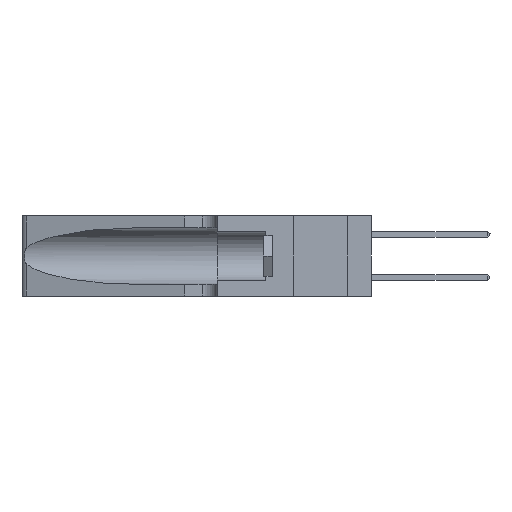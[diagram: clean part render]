
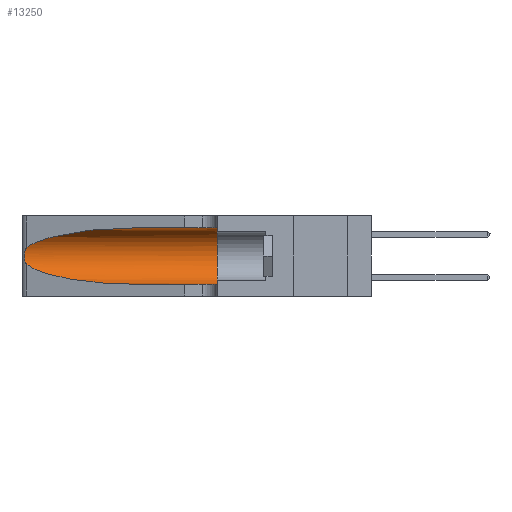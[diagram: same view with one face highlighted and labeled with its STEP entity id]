
A CAD part, left-side view. The second image highlights one B-rep face of the part: STEP entity #13250.
In plain terms, the highlighted cylindrical face has radius 3.308 mm (diameter 6.617 mm), a partial arc.
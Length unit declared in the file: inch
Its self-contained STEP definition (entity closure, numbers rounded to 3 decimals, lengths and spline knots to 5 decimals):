
#466 = DIRECTION ( 'NONE',  ( 0., -1., 0. ) ) ;
#1158 = CARTESIAN_POINT ( 'NONE',  ( 0.26018, 1.23835, 0.19895 ) ) ;
#1404 = CARTESIAN_POINT ( 'NONE',  ( 0.25487, 1.22718, 0.22369 ) ) ;
#1610 = ORIENTED_EDGE ( 'NONE', *, *, #1614, .F. ) ;
#1614 = EDGE_CURVE ( 'NONE', #12219, #10811, #5486, .T. ) ;
#2784 = VERTEX_POINT ( 'NONE', #10919 ) ;
#3236 = VERTEX_POINT ( 'NONE', #11997 ) ;
#4384 = EDGE_CURVE ( 'NONE', #2784, #16755, #19624, .T. ) ;
#5141 = DIRECTION ( 'NONE',  ( 0., 0., -1. ) ) ;
#5486 = CIRCLE ( 'NONE', #8405, 0.13025 ) ;
#5606 = CARTESIAN_POINT ( 'NONE',  ( 0.26017, 1.23833, 0.17102 ) ) ;
#5925 = CARTESIAN_POINT ( 'NONE',  ( 0.1305, 0.72297, 0.31525 ) ) ;
#6008 = ORIENTED_EDGE ( 'NONE', *, *, #16518, .T. ) ;
#6094 = CARTESIAN_POINT ( 'NONE',  ( 0.1305, 0.35, 0.05475 ) ) ;
#6561 = DIRECTION ( 'NONE',  ( 0., -1., 0. ) ) ;
#6640 = CARTESIAN_POINT ( 'NONE',  ( 0.1305, 0.72297, 0.05475 ) ) ;
#7011 = CARTESIAN_POINT ( 'NONE',  ( 0.25639, 1.23184, 0.21858 ) ) ;
#7334 = CARTESIAN_POINT ( 'NONE',  ( 0.26075, 1.23896, 0.178 ) ) ;
#7349 = DIRECTION ( 'NONE',  ( 0., 1., 0. ) ) ;
#7980 = VERTEX_POINT ( 'NONE', #5925 ) ;
#8367 = EDGE_CURVE ( 'NONE', #7980, #3236, #24157, .T. ) ;
#8405 = AXIS2_PLACEMENT_3D ( 'NONE', #18432, #7349, #14829 ) ;
#8861 = CARTESIAN_POINT ( 'NONE',  ( 0.25787, 1.23484, 0.2124 ) ) ;
#8990 = VECTOR ( 'NONE', #466, 39.37008 ) ;
#9025 = CARTESIAN_POINT ( 'NONE',  ( 0.25854, 1.2359, 0.20912 ) ) ;
#9101 = CARTESIAN_POINT ( 'NONE',  ( 0.18966, 0.96281, 0.31525 ) ) ;
#9102 = CARTESIAN_POINT ( 'NONE',  ( 0.1305, 0.72297, 0.05475 ) ) ;
#9343 = CARTESIAN_POINT ( 'NONE',  ( 0.1305, 0.35, 0.31525 ) ) ;
#9412 = CARTESIAN_POINT ( 'NONE',  ( 0.1305, 1.61858, 0.31525 ) ) ;
#10445 = CYLINDRICAL_SURFACE ( 'NONE', #16568, 0.13025 ) ;
#10811 = VERTEX_POINT ( 'NONE', #6094 ) ;
#10896 = CARTESIAN_POINT ( 'NONE',  ( 0.25639, 1.23186, 0.15144 ) ) ;
#10919 = CARTESIAN_POINT ( 'NONE',  ( 0.25487, 1.22718, 0.14631 ) ) ;
#11144 = CARTESIAN_POINT ( 'NONE',  ( 0.25487, 1.22718, 0.14631 ) ) ;
#11997 = CARTESIAN_POINT ( 'NONE',  ( 0.25487, 1.22718, 0.22369 ) ) ;
#12219 = VERTEX_POINT ( 'NONE', #9343 ) ;
#12611 = ORIENTED_EDGE ( 'NONE', *, *, #4384, .T. ) ;
#13250 = ADVANCED_FACE ( 'NONE', ( #23665 ), #10445, .F. ) ;
#13272 = VECTOR ( 'NONE', #6561, 39.37008 ) ;
#13796 = EDGE_CURVE ( 'NONE', #7980, #12219, #17737, .T. ) ;
#14435 = DIRECTION ( 'NONE',  ( 0., -1., 0. ) ) ;
#14829 = DIRECTION ( 'NONE',  ( 0., 0., 1. ) ) ;
#15478 = EDGE_LOOP ( 'NONE', ( #19360, #23153, #12611, #6008, #1610, #18938 ) ) ;
#15530 = EDGE_CURVE ( 'NONE', #3236, #2784, #19344, .T. ) ;
#15871 = LINE ( 'NONE', #17646, #13272 ) ;
#16518 = EDGE_CURVE ( 'NONE', #16755, #10811, #15871, .T. ) ;
#16568 = AXIS2_PLACEMENT_3D ( 'NONE', #23865, #14435, #5141 ) ;
#16755 = VERTEX_POINT ( 'NONE', #9102 ) ;
#17646 = CARTESIAN_POINT ( 'NONE',  ( 0.1305, 1.61858, 0.05475 ) ) ;
#17737 = LINE ( 'NONE', #9412, #8990 ) ;
#17999 = CARTESIAN_POINT ( 'NONE',  ( 0.25555, 1.22994, 0.2215 ) ) ;
#18161 = CARTESIAN_POINT ( 'NONE',  ( 0.1305, 0.72297, 0.31525 ) ) ;
#18432 = CARTESIAN_POINT ( 'NONE',  ( 0.1305, 0.35, 0.185 ) ) ;
#18938 = ORIENTED_EDGE ( 'NONE', *, *, #13796, .F. ) ;
#19344 = B_SPLINE_CURVE_WITH_KNOTS ( 'NONE', 3,
 ( #22018, #17999, #7011, #8861, #9025, #1158, #19910, #7334, #5606, #20402, #22348, #10896, #23800, #11144 ),
 .UNSPECIFIED., .F., .F.,
 ( 4, 2, 2, 2, 2, 2, 4 ),
 ( 0., 0.00027, 0.00053, 0.00107, 0.0016, 0.00187, 0.00214 ),
 .UNSPECIFIED. ) ;
#19360 = ORIENTED_EDGE ( 'NONE', *, *, #8367, .T. ) ;
#19624 =( BOUNDED_CURVE ( )  B_SPLINE_CURVE ( 3, ( #23330, #21512, #19707, #6640 ),
 .UNSPECIFIED., .F., .T. ) 
 B_SPLINE_CURVE_WITH_KNOTS ( ( 4, 4 ),
 ( 3.44316, 4.71239 ),
 .UNSPECIFIED. ) 
 CURVE ( )  GEOMETRIC_REPRESENTATION_ITEM ( )  RATIONAL_B_SPLINE_CURVE ( ( 1., 0.87, 0.87, 1. ) ) 
 REPRESENTATION_ITEM ( '' )  );
#19707 = CARTESIAN_POINT ( 'NONE',  ( 0.18966, 0.96281, 0.05475 ) ) ;
#19910 = CARTESIAN_POINT ( 'NONE',  ( 0.26075, 1.23896, 0.19203 ) ) ;
#19992 = CARTESIAN_POINT ( 'NONE',  ( 0.2373, 1.15595, 0.28018 ) ) ;
#20402 = CARTESIAN_POINT ( 'NONE',  ( 0.25856, 1.23593, 0.16098 ) ) ;
#21512 = CARTESIAN_POINT ( 'NONE',  ( 0.2373, 1.15595, 0.08982 ) ) ;
#22018 = CARTESIAN_POINT ( 'NONE',  ( 0.25487, 1.22718, 0.22369 ) ) ;
#22348 = CARTESIAN_POINT ( 'NONE',  ( 0.25789, 1.23486, 0.15765 ) ) ;
#23153 = ORIENTED_EDGE ( 'NONE', *, *, #15530, .T. ) ;
#23330 = CARTESIAN_POINT ( 'NONE',  ( 0.25487, 1.22718, 0.14631 ) ) ;
#23665 = FACE_OUTER_BOUND ( 'NONE', #15478, .T. ) ;
#23800 = CARTESIAN_POINT ( 'NONE',  ( 0.25555, 1.22993, 0.14849 ) ) ;
#23865 = CARTESIAN_POINT ( 'NONE',  ( 0.1305, 1.61858, 0.185 ) ) ;
#24157 =( BOUNDED_CURVE ( )  B_SPLINE_CURVE ( 3, ( #18161, #9101, #19992, #1404 ),
 .UNSPECIFIED., .F., .T. ) 
 B_SPLINE_CURVE_WITH_KNOTS ( ( 4, 4 ),
 ( 1.5708, 2.84003 ),
 .UNSPECIFIED. ) 
 CURVE ( )  GEOMETRIC_REPRESENTATION_ITEM ( )  RATIONAL_B_SPLINE_CURVE ( ( 1., 0.87, 0.87, 1. ) ) 
 REPRESENTATION_ITEM ( '' )  );
